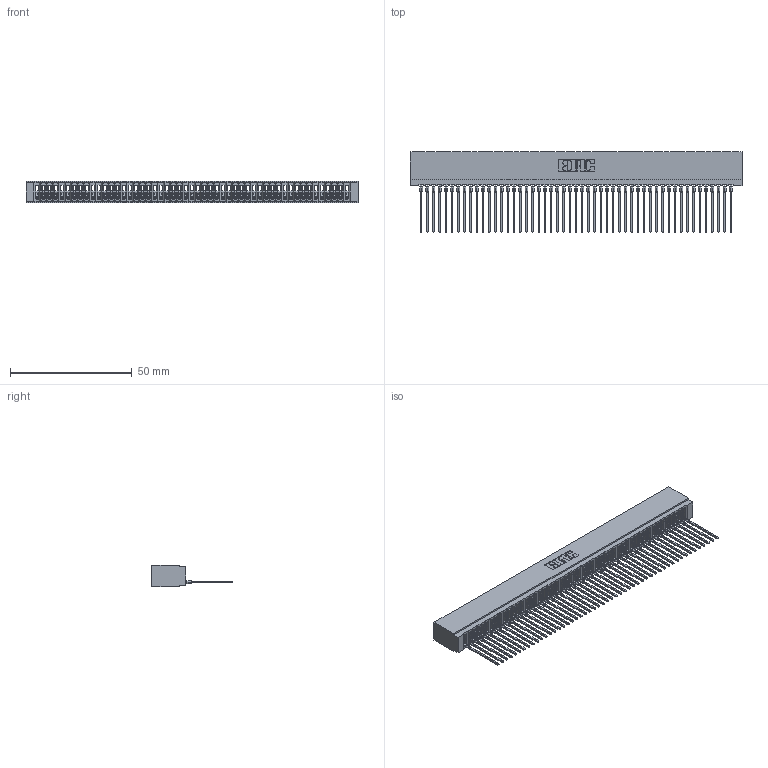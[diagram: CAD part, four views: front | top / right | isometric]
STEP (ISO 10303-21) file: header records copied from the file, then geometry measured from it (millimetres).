
FILE_DESCRIPTION (( 'STEP AP203' ), '1' );
FILE_NAME ('725-051-541-101.STEP', '2020-09-10T00:38:28', ( '' ), ( '' ), 'SwSTEP 2.0', 'SolidWorks 2020', '' );
FILE_SCHEMA (( 'CONFIG_CONTROL_DESIGN' ));
Products named in the file (3): 725 Part_Insulator Option - 01; 725-051-541-101; 745-292-001_541
Assembly tree (52 placements, depth 2):
  725-051-541-101
    725 Part_Insulator Option - 01
    745-292-001_541  x51
Bounding box: 136.14 x 33.03 x 8.89 mm (x, y, z)
Volume: 10501.3 mm3; surface area: 21365 mm2
Topology: 52 solids, 52 shells, 5807 faces, 15962 edges, 10062 vertices
Faces by surface type: plane 3472, bspline 1020, cylinder 1009, torus 306
Entity records: 82969 total; most frequent: CARTESIAN_POINT 15120, ORIENTED_EDGE 14624, DIRECTION 12668, EDGE_CURVE 7312, LINE 6824, VECTOR 6824, VERTEX_POINT 4662, AXIS2_PLACEMENT_3D 2922
